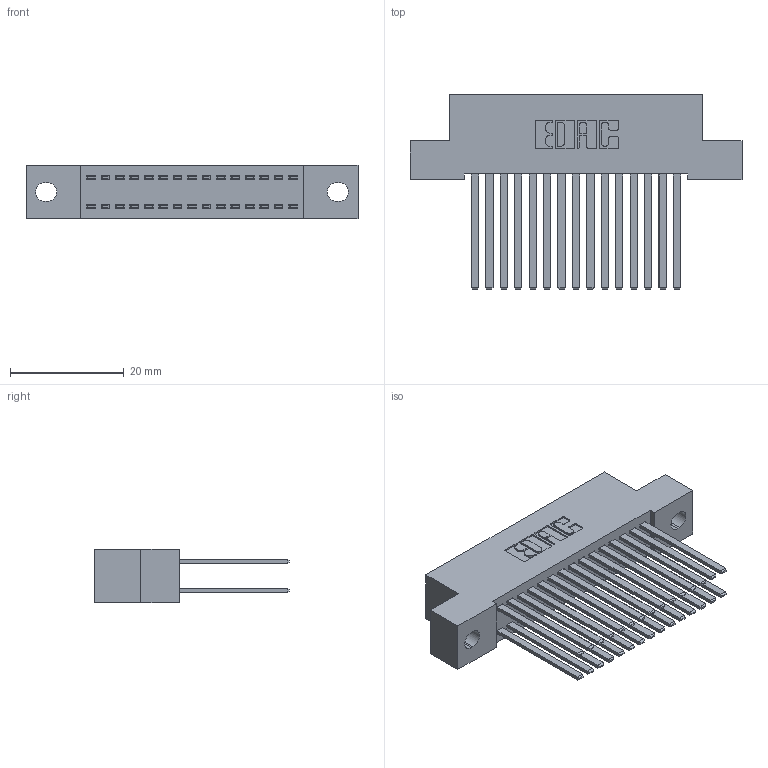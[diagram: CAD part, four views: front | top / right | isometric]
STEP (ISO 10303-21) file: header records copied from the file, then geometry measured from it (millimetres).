
FILE_DESCRIPTION (( 'STEP AP203' ), '1' );
FILE_NAME ('342-030-544-202.STEP', '2018-08-11T15:43:22', ( '' ), ( '' ), 'SwSTEP 2.0', 'SolidWorks 2016', '' );
FILE_SCHEMA (( 'CONFIG_CONTROL_DESIGN' ));
Length unit declared in the file: inch
Products named in the file (3): 342 Part_.128 Slot; 345-292-001_345-293-144; 342-030-544-202
Assembly tree (31 placements, depth 2):
  342-030-544-202
    342 Part_.128 Slot
    345-292-001_345-293-144  x30
Bounding box: 58.42 x 34.3 x 9.4 mm (x, y, z)
Volume: 5489.6 mm3; surface area: 9194.6 mm2
Topology: 31 solids, 31 shells, 1494 faces, 4421 edges, 2906 vertices
Faces by surface type: plane 1030, cylinder 464
Entity records: 12961 total; most frequent: CARTESIAN_POINT 2178, ORIENTED_EDGE 2114, DIRECTION 1905, EDGE_CURVE 1057, VECTOR 933, LINE 933, VERTEX_POINT 702, AXIS2_PLACEMENT_3D 486
